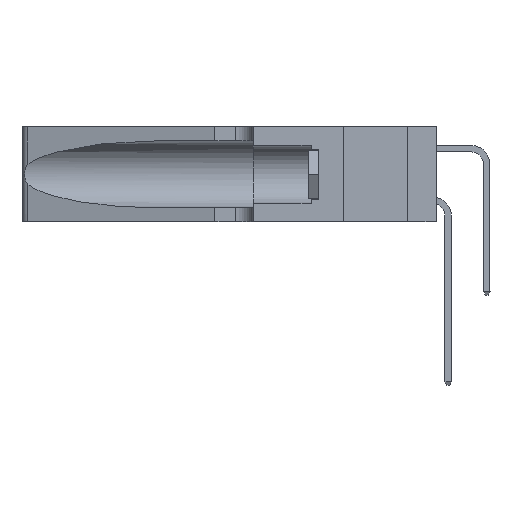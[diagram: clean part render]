
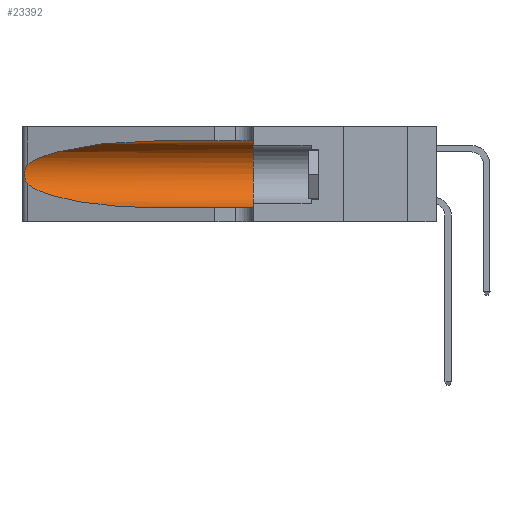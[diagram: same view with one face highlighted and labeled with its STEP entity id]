
A CAD part, left-side view. The second image highlights one B-rep face of the part: STEP entity #23392.
In plain terms, the highlighted cylindrical face has radius 3.308 mm (diameter 6.617 mm), a partial arc.
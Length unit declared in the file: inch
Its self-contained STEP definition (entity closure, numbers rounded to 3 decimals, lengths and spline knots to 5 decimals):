
#68 = CARTESIAN_POINT ( 'NONE',  ( 0.25555, 1.22993, 0.14849 ) ) ;
#280 = ORIENTED_EDGE ( 'NONE', *, *, #15092, .F. ) ;
#319 = CARTESIAN_POINT ( 'NONE',  ( 0.25487, 1.22718, 0.14631 ) ) ;
#1375 = ORIENTED_EDGE ( 'NONE', *, *, #3275, .F. ) ;
#1716 = B_SPLINE_CURVE_WITH_KNOTS ( 'NONE', 3,
 ( #8619, #2945, #20075, #18077, #8796, #6795, #14735, #10921, #3433, #10847, #16495, #22391, #68, #319 ),
 .UNSPECIFIED., .F., .F.,
 ( 4, 2, 2, 2, 2, 2, 4 ),
 ( 0., 0.00027, 0.00053, 0.00107, 0.0016, 0.00187, 0.00214 ),
 .UNSPECIFIED. ) ;
#1765 = LINE ( 'NONE', #12964, #18626 ) ;
#2712 = EDGE_LOOP ( 'NONE', ( #6176, #22634, #12807, #14180, #1375, #280 ) ) ;
#2945 = CARTESIAN_POINT ( 'NONE',  ( 0.25555, 1.22994, 0.2215 ) ) ;
#3275 = EDGE_CURVE ( 'NONE', #12047, #18620, #19909, .T. ) ;
#3433 = CARTESIAN_POINT ( 'NONE',  ( 0.26017, 1.23833, 0.17102 ) ) ;
#3569 = DIRECTION ( 'NONE',  ( 0., 1., 0. ) ) ;
#3850 = CARTESIAN_POINT ( 'NONE',  ( 0.18966, 0.96281, 0.31525 ) ) ;
#3934 = VERTEX_POINT ( 'NONE', #7403 ) ;
#3960 = EDGE_CURVE ( 'NONE', #3934, #9493, #1716, .T. ) ;
#3987 =( BOUNDED_CURVE ( )  B_SPLINE_CURVE ( 3, ( #11099, #3850, #7698, #9286 ),
 .UNSPECIFIED., .F., .T. ) 
 B_SPLINE_CURVE_WITH_KNOTS ( ( 4, 4 ),
 ( 1.5708, 2.84003 ),
 .UNSPECIFIED. ) 
 CURVE ( )  GEOMETRIC_REPRESENTATION_ITEM ( )  RATIONAL_B_SPLINE_CURVE ( ( 1., 0.87, 0.87, 1. ) ) 
 REPRESENTATION_ITEM ( '' )  );
#6176 = ORIENTED_EDGE ( 'NONE', *, *, #12271, .T. ) ;
#6795 = CARTESIAN_POINT ( 'NONE',  ( 0.26018, 1.23835, 0.19895 ) ) ;
#7403 = CARTESIAN_POINT ( 'NONE',  ( 0.25487, 1.22718, 0.22369 ) ) ;
#7698 = CARTESIAN_POINT ( 'NONE',  ( 0.2373, 1.15595, 0.28018 ) ) ;
#7917 = CARTESIAN_POINT ( 'NONE',  ( 0.1305, 0.72297, 0.31525 ) ) ;
#8619 = CARTESIAN_POINT ( 'NONE',  ( 0.25487, 1.22718, 0.22369 ) ) ;
#8796 = CARTESIAN_POINT ( 'NONE',  ( 0.25854, 1.2359, 0.20912 ) ) ;
#9286 = CARTESIAN_POINT ( 'NONE',  ( 0.25487, 1.22718, 0.22369 ) ) ;
#9493 = VERTEX_POINT ( 'NONE', #14303 ) ;
#9786 = VERTEX_POINT ( 'NONE', #12757 ) ;
#9945 = CARTESIAN_POINT ( 'NONE',  ( 0.1305, 1.61858, 0.05475 ) ) ;
#10847 = CARTESIAN_POINT ( 'NONE',  ( 0.25856, 1.23593, 0.16098 ) ) ;
#10921 = CARTESIAN_POINT ( 'NONE',  ( 0.26075, 1.23896, 0.178 ) ) ;
#11053 = EDGE_CURVE ( 'NONE', #9493, #9786, #15648, .T. ) ;
#11074 = AXIS2_PLACEMENT_3D ( 'NONE', #13097, #11253, #17207 ) ;
#11099 = CARTESIAN_POINT ( 'NONE',  ( 0.1305, 0.72297, 0.31525 ) ) ;
#11253 = DIRECTION ( 'NONE',  ( 0., -1., 0. ) ) ;
#12047 = VERTEX_POINT ( 'NONE', #12051 ) ;
#12051 = CARTESIAN_POINT ( 'NONE',  ( 0.1305, 0.35, 0.31525 ) ) ;
#12271 = EDGE_CURVE ( 'NONE', #12713, #3934, #3987, .T. ) ;
#12713 = VERTEX_POINT ( 'NONE', #7917 ) ;
#12757 = CARTESIAN_POINT ( 'NONE',  ( 0.1305, 0.72297, 0.05475 ) ) ;
#12807 = ORIENTED_EDGE ( 'NONE', *, *, #11053, .T. ) ;
#12964 = CARTESIAN_POINT ( 'NONE',  ( 0.1305, 1.61858, 0.31525 ) ) ;
#12987 = DIRECTION ( 'NONE',  ( 0., 0., 1. ) ) ;
#13097 = CARTESIAN_POINT ( 'NONE',  ( 0.1305, 1.61858, 0.185 ) ) ;
#14180 = ORIENTED_EDGE ( 'NONE', *, *, #22785, .T. ) ;
#14222 = CARTESIAN_POINT ( 'NONE',  ( 0.25487, 1.22718, 0.14631 ) ) ;
#14303 = CARTESIAN_POINT ( 'NONE',  ( 0.25487, 1.22718, 0.14631 ) ) ;
#14735 = CARTESIAN_POINT ( 'NONE',  ( 0.26075, 1.23896, 0.19203 ) ) ;
#15092 = EDGE_CURVE ( 'NONE', #12713, #12047, #1765, .T. ) ;
#15187 = CARTESIAN_POINT ( 'NONE',  ( 0.1305, 0.35, 0.185 ) ) ;
#15648 =( BOUNDED_CURVE ( )  B_SPLINE_CURVE ( 3, ( #14222, #20043, #17964, #24048 ),
 .UNSPECIFIED., .F., .F. ) 
 B_SPLINE_CURVE_WITH_KNOTS ( ( 4, 4 ),
 ( 3.44316, 4.71239 ),
 .UNSPECIFIED. ) 
 CURVE ( )  GEOMETRIC_REPRESENTATION_ITEM ( )  RATIONAL_B_SPLINE_CURVE ( ( 1., 0.87, 0.87, 1. ) ) 
 REPRESENTATION_ITEM ( '' )  );
#16379 = AXIS2_PLACEMENT_3D ( 'NONE', #15187, #3569, #12987 ) ;
#16495 = CARTESIAN_POINT ( 'NONE',  ( 0.25789, 1.23486, 0.15765 ) ) ;
#16840 = DIRECTION ( 'NONE',  ( 0., -1., 0. ) ) ;
#17207 = DIRECTION ( 'NONE',  ( 0., 0., -1. ) ) ;
#17964 = CARTESIAN_POINT ( 'NONE',  ( 0.18966, 0.96281, 0.05475 ) ) ;
#18077 = CARTESIAN_POINT ( 'NONE',  ( 0.25787, 1.23484, 0.2124 ) ) ;
#18620 = VERTEX_POINT ( 'NONE', #19179 ) ;
#18626 = VECTOR ( 'NONE', #16840, 39.37008 ) ;
#19179 = CARTESIAN_POINT ( 'NONE',  ( 0.1305, 0.35, 0.05475 ) ) ;
#19597 = LINE ( 'NONE', #9945, #24388 ) ;
#19909 = CIRCLE ( 'NONE', #16379, 0.13025 ) ;
#20043 = CARTESIAN_POINT ( 'NONE',  ( 0.2373, 1.15595, 0.08982 ) ) ;
#20075 = CARTESIAN_POINT ( 'NONE',  ( 0.25639, 1.23184, 0.21858 ) ) ;
#22391 = CARTESIAN_POINT ( 'NONE',  ( 0.25639, 1.23186, 0.15144 ) ) ;
#22542 = CYLINDRICAL_SURFACE ( 'NONE', #11074, 0.13025 ) ;
#22634 = ORIENTED_EDGE ( 'NONE', *, *, #3960, .T. ) ;
#22785 = EDGE_CURVE ( 'NONE', #9786, #18620, #19597, .T. ) ;
#22985 = DIRECTION ( 'NONE',  ( 0., -1., 0. ) ) ;
#23126 = FACE_OUTER_BOUND ( 'NONE', #2712, .T. ) ;
#23392 = ADVANCED_FACE ( 'NONE', ( #23126 ), #22542, .F. ) ;
#24048 = CARTESIAN_POINT ( 'NONE',  ( 0.1305, 0.72297, 0.05475 ) ) ;
#24388 = VECTOR ( 'NONE', #22985, 39.37008 ) ;
